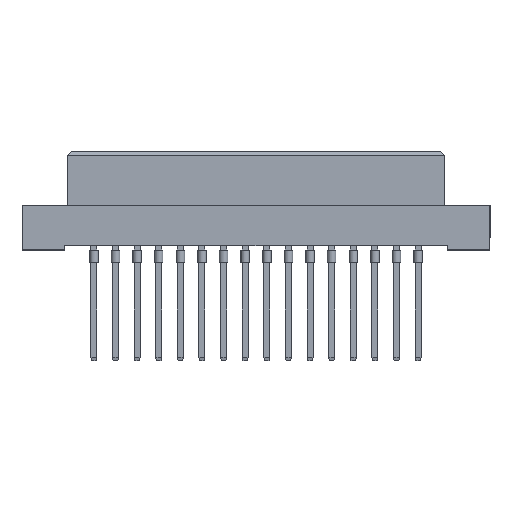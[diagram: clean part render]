
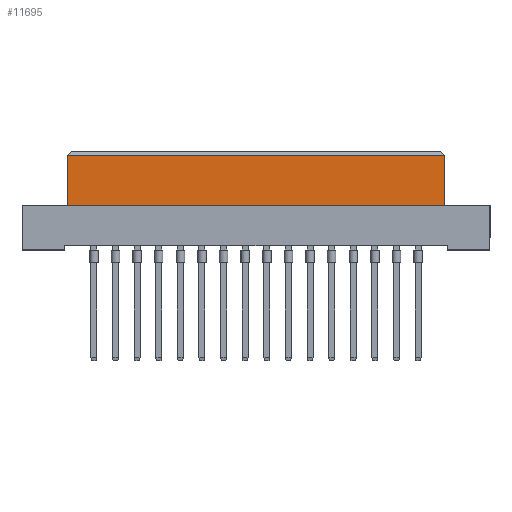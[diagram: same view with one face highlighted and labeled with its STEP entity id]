
A CAD part, top view. The second image highlights one B-rep face of the part: STEP entity #11695.
In plain terms, the highlighted planar face has unit normal (0, 0, 1).
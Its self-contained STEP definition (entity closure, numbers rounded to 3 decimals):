
#215 = VERTEX_POINT ( 'NONE', #1610 ) ;
#1190 = VECTOR ( 'NONE', #16521, 1000. ) ;
#1610 = CARTESIAN_POINT ( 'NONE',  ( 22.2, -0.5, 4.25 ) ) ;
#2208 = ORIENTED_EDGE ( 'NONE', *, *, #9047, .T. ) ;
#3552 = LINE ( 'NONE', #10050, #1190 ) ;
#4041 = VECTOR ( 'NONE', #9649, 1000. ) ;
#4623 = EDGE_CURVE ( 'NONE', #15781, #20101, #3552, .T. ) ;
#5526 = CARTESIAN_POINT ( 'NONE',  ( -22.2, -6.4, 4.25 ) ) ;
#6569 = CARTESIAN_POINT ( 'NONE',  ( -22.2, -0.5, 4.25 ) ) ;
#6895 = CARTESIAN_POINT ( 'NONE',  ( -22.2, -0.5, 4.25 ) ) ;
#6986 = CARTESIAN_POINT ( 'NONE',  ( 22.2, -6.4, 4.25 ) ) ;
#7145 = ORIENTED_EDGE ( 'NONE', *, *, #4623, .T. ) ;
#7624 = EDGE_LOOP ( 'NONE', ( #2208, #18112, #15635, #7145 ) ) ;
#7856 = CARTESIAN_POINT ( 'NONE',  ( 22.2, -6.4, 4.25 ) ) ;
#8177 = PLANE ( 'NONE',  #9109 ) ;
#9047 = EDGE_CURVE ( 'NONE', #20101, #215, #17638, .T. ) ;
#9109 = AXIS2_PLACEMENT_3D ( 'NONE', #16657, #16760, #9974 ) ;
#9325 = FACE_OUTER_BOUND ( 'NONE', #7624, .T. ) ;
#9649 = DIRECTION ( 'NONE',  ( 0., 1., 0. ) ) ;
#9974 = DIRECTION ( 'NONE',  ( 1., 0., 0. ) ) ;
#10050 = CARTESIAN_POINT ( 'NONE',  ( 22.2, -6.4, 4.25 ) ) ;
#11695 = ADVANCED_FACE ( 'NONE', ( #9325 ), #8177, .T. ) ;
#13192 = LINE ( 'NONE', #6895, #18497 ) ;
#14294 = VERTEX_POINT ( 'NONE', #6569 ) ;
#15635 = ORIENTED_EDGE ( 'NONE', *, *, #20407, .F. ) ;
#15781 = VERTEX_POINT ( 'NONE', #5526 ) ;
#16328 = LINE ( 'NONE', #16423, #20196 ) ;
#16366 = DIRECTION ( 'NONE',  ( -1., 0., 0. ) ) ;
#16423 = CARTESIAN_POINT ( 'NONE',  ( -22.2, -6.4, 4.25 ) ) ;
#16521 = DIRECTION ( 'NONE',  ( 1., 0., 0. ) ) ;
#16657 = CARTESIAN_POINT ( 'NONE',  ( 22.2, -6.4, 4.25 ) ) ;
#16760 = DIRECTION ( 'NONE',  ( 0., 0., 1. ) ) ;
#17638 = LINE ( 'NONE', #7856, #4041 ) ;
#18112 = ORIENTED_EDGE ( 'NONE', *, *, #20716, .T. ) ;
#18497 = VECTOR ( 'NONE', #16366, 1000. ) ;
#19415 = DIRECTION ( 'NONE',  ( 0., 1., 0. ) ) ;
#20101 = VERTEX_POINT ( 'NONE', #6986 ) ;
#20196 = VECTOR ( 'NONE', #19415, 1000. ) ;
#20407 = EDGE_CURVE ( 'NONE', #15781, #14294, #16328, .T. ) ;
#20716 = EDGE_CURVE ( 'NONE', #215, #14294, #13192, .T. ) ;
